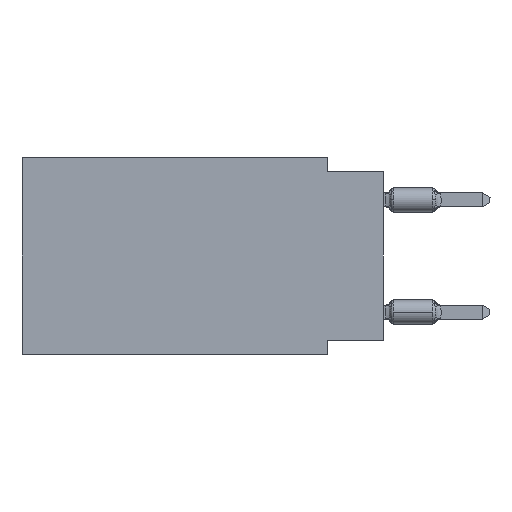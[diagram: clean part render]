
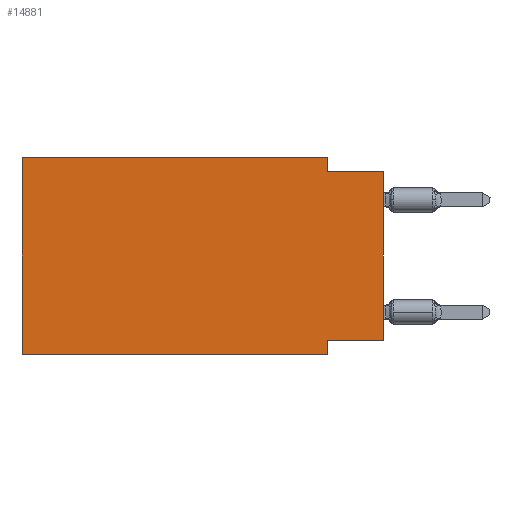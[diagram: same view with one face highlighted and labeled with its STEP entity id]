
A CAD part, left-side view. The second image highlights one B-rep face of the part: STEP entity #14881.
In plain terms, the highlighted planar face has unit normal (-1, 0, 0).
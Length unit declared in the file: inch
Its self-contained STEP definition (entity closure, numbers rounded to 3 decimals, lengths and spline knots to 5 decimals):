
#112 = EDGE_CURVE ( 'NONE', #11930, #10315, #22014, .T. ) ;
#347 = CARTESIAN_POINT ( 'NONE',  ( 0., 0.1, 0. ) ) ;
#365 = LINE ( 'NONE', #29062, #12589 ) ;
#1177 = VECTOR ( 'NONE', #15241, 39.37008 ) ;
#1743 = CARTESIAN_POINT ( 'NONE',  ( 0., 0., -0.025 ) ) ;
#2222 = CARTESIAN_POINT ( 'NONE',  ( 0., 0.645, 0. ) ) ;
#2610 = ORIENTED_EDGE ( 'NONE', *, *, #12833, .F. ) ;
#3391 = LINE ( 'NONE', #10618, #10847 ) ;
#3793 = VERTEX_POINT ( 'NONE', #26891 ) ;
#4552 = DIRECTION ( 'NONE',  ( 0., -1., 0. ) ) ;
#5098 = ORIENTED_EDGE ( 'NONE', *, *, #13935, .T. ) ;
#5796 = EDGE_CURVE ( 'NONE', #3793, #28986, #12737, .T. ) ;
#6068 = VECTOR ( 'NONE', #19774, 39.37008 ) ;
#6401 = CARTESIAN_POINT ( 'NONE',  ( 0., 0.1, -0.35 ) ) ;
#7254 = CARTESIAN_POINT ( 'NONE',  ( 0., 0.645, 0. ) ) ;
#8381 = ORIENTED_EDGE ( 'NONE', *, *, #10353, .F. ) ;
#9330 = ORIENTED_EDGE ( 'NONE', *, *, #28203, .F. ) ;
#9411 = FACE_OUTER_BOUND ( 'NONE', #9609, .T. ) ;
#9609 = EDGE_LOOP ( 'NONE', ( #17570, #8381, #24636, #9330, #29770, #5098, #17878, #2610 ) ) ;
#9863 = PLANE ( 'NONE',  #17925 ) ;
#10315 = VERTEX_POINT ( 'NONE', #7254 ) ;
#10353 = EDGE_CURVE ( 'NONE', #28986, #24227, #29202, .T. ) ;
#10618 = CARTESIAN_POINT ( 'NONE',  ( 0., 0., 0. ) ) ;
#10847 = VECTOR ( 'NONE', #12961, 39.37008 ) ;
#11821 = CARTESIAN_POINT ( 'NONE',  ( 0., 0., -0.325 ) ) ;
#11930 = VERTEX_POINT ( 'NONE', #29013 ) ;
#12589 = VECTOR ( 'NONE', #14647, 39.37008 ) ;
#12737 = LINE ( 'NONE', #347, #21096 ) ;
#12833 = EDGE_CURVE ( 'NONE', #23432, #30496, #23194, .T. ) ;
#12961 = DIRECTION ( 'NONE',  ( 0., 0., 1. ) ) ;
#13736 = CARTESIAN_POINT ( 'NONE',  ( 0., 0.1, -0.325 ) ) ;
#13935 = EDGE_CURVE ( 'NONE', #11930, #21270, #15100, .T. ) ;
#14433 = VECTOR ( 'NONE', #15555, 39.37008 ) ;
#14464 = DIRECTION ( 'NONE',  ( 0., -1., 0. ) ) ;
#14636 = CARTESIAN_POINT ( 'NONE',  ( 0., 0.645, -0.35 ) ) ;
#14647 = DIRECTION ( 'NONE',  ( 0., 0., -1. ) ) ;
#14881 = ADVANCED_FACE ( 'NONE', ( #9411 ), #9863, .F. ) ;
#15100 = LINE ( 'NONE', #14636, #20681 ) ;
#15241 = DIRECTION ( 'NONE',  ( 0., 1., 0. ) ) ;
#15555 = DIRECTION ( 'NONE',  ( 0., 0., 1. ) ) ;
#17278 = CARTESIAN_POINT ( 'NONE',  ( 0., 0., -0.025 ) ) ;
#17570 = ORIENTED_EDGE ( 'NONE', *, *, #21779, .T. ) ;
#17878 = ORIENTED_EDGE ( 'NONE', *, *, #18259, .F. ) ;
#17925 = AXIS2_PLACEMENT_3D ( 'NONE', #2222, #23539, #19432 ) ;
#18259 = EDGE_CURVE ( 'NONE', #30496, #21270, #365, .T. ) ;
#19432 = DIRECTION ( 'NONE',  ( 0., 0., -1. ) ) ;
#19774 = DIRECTION ( 'NONE',  ( 0., -1., 0. ) ) ;
#20681 = VECTOR ( 'NONE', #14464, 39.37008 ) ;
#21096 = VECTOR ( 'NONE', #22280, 39.37008 ) ;
#21179 = LINE ( 'NONE', #23526, #26396 ) ;
#21270 = VERTEX_POINT ( 'NONE', #6401 ) ;
#21779 = EDGE_CURVE ( 'NONE', #23432, #24227, #3391, .T. ) ;
#22014 = LINE ( 'NONE', #26719, #14433 ) ;
#22280 = DIRECTION ( 'NONE',  ( 0., 0., -1. ) ) ;
#23194 = LINE ( 'NONE', #27154, #1177 ) ;
#23432 = VERTEX_POINT ( 'NONE', #11821 ) ;
#23526 = CARTESIAN_POINT ( 'NONE',  ( 0., 0.645, 0. ) ) ;
#23539 = DIRECTION ( 'NONE',  ( 1., 0., 0. ) ) ;
#24132 = CARTESIAN_POINT ( 'NONE',  ( 0., 0.1, -0.025 ) ) ;
#24227 = VERTEX_POINT ( 'NONE', #1743 ) ;
#24636 = ORIENTED_EDGE ( 'NONE', *, *, #5796, .F. ) ;
#26396 = VECTOR ( 'NONE', #4552, 39.37008 ) ;
#26719 = CARTESIAN_POINT ( 'NONE',  ( 0., 0.645, 0. ) ) ;
#26891 = CARTESIAN_POINT ( 'NONE',  ( 0., 0.1, 0. ) ) ;
#27154 = CARTESIAN_POINT ( 'NONE',  ( 0., 0., -0.325 ) ) ;
#28203 = EDGE_CURVE ( 'NONE', #10315, #3793, #21179, .T. ) ;
#28986 = VERTEX_POINT ( 'NONE', #24132 ) ;
#29013 = CARTESIAN_POINT ( 'NONE',  ( 0., 0.645, -0.35 ) ) ;
#29062 = CARTESIAN_POINT ( 'NONE',  ( 0., 0.1, -0.35 ) ) ;
#29202 = LINE ( 'NONE', #17278, #6068 ) ;
#29770 = ORIENTED_EDGE ( 'NONE', *, *, #112, .F. ) ;
#30496 = VERTEX_POINT ( 'NONE', #13736 ) ;
